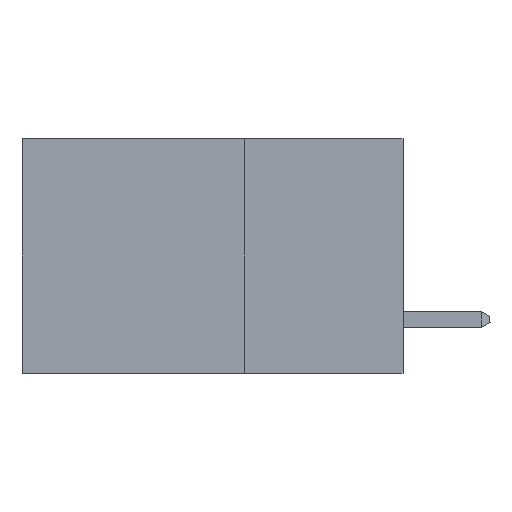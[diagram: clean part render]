
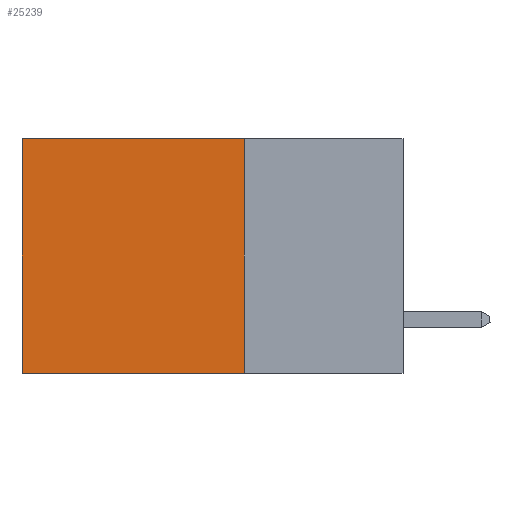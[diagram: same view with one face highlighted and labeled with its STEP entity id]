
A CAD part, left-side view. The second image highlights one B-rep face of the part: STEP entity #25239.
In plain terms, the highlighted planar face has unit normal (-1, 0, 0).
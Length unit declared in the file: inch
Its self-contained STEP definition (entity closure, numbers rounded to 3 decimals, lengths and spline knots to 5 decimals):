
#1947 = CARTESIAN_POINT ( 'NONE',  ( 0.2875, 0.25, 0. ) ) ;
#2857 = DIRECTION ( 'NONE',  ( 0., 1., 0. ) ) ;
#2912 = ORIENTED_EDGE ( 'NONE', *, *, #10901, .F. ) ;
#4572 = VECTOR ( 'NONE', #8543, 39.37008 ) ;
#4784 = VECTOR ( 'NONE', #24970, 39.37008 ) ;
#5266 = VERTEX_POINT ( 'NONE', #1947 ) ;
#7312 = LINE ( 'NONE', #16589, #4784 ) ;
#8152 = EDGE_CURVE ( 'NONE', #25334, #18882, #29301, .T. ) ;
#8543 = DIRECTION ( 'NONE',  ( 0., 0., -1. ) ) ;
#9494 = EDGE_LOOP ( 'NONE', ( #34622, #2912, #14460, #10343 ) ) ;
#10343 = ORIENTED_EDGE ( 'NONE', *, *, #18766, .T. ) ;
#10901 = EDGE_CURVE ( 'NONE', #11568, #18882, #7312, .T. ) ;
#11568 = VERTEX_POINT ( 'NONE', #30639 ) ;
#12068 = DIRECTION ( 'NONE',  ( 0., 0., -1. ) ) ;
#12551 = PLANE ( 'NONE',  #35012 ) ;
#14402 = LINE ( 'NONE', #19249, #26872 ) ;
#14460 = ORIENTED_EDGE ( 'NONE', *, *, #15959, .F. ) ;
#15959 = EDGE_CURVE ( 'NONE', #5266, #11568, #29361, .T. ) ;
#16589 = CARTESIAN_POINT ( 'NONE',  ( 0.2875, 0.25, -0.37 ) ) ;
#17227 = CARTESIAN_POINT ( 'NONE',  ( 0.2875, 0.25, 0. ) ) ;
#17566 = CARTESIAN_POINT ( 'NONE',  ( 0.2875, 0.25, 0. ) ) ;
#17691 = CARTESIAN_POINT ( 'NONE',  ( 0.2875, 0.6, 0. ) ) ;
#18717 = VECTOR ( 'NONE', #33597, 39.37008 ) ;
#18766 = EDGE_CURVE ( 'NONE', #5266, #25334, #14402, .T. ) ;
#18882 = VERTEX_POINT ( 'NONE', #34020 ) ;
#19249 = CARTESIAN_POINT ( 'NONE',  ( 0.2875, 0.25, 0. ) ) ;
#19938 = CARTESIAN_POINT ( 'NONE',  ( 0.2875, 0.6, 0. ) ) ;
#22181 = FACE_OUTER_BOUND ( 'NONE', #9494, .T. ) ;
#24970 = DIRECTION ( 'NONE',  ( 0., 1., 0. ) ) ;
#25239 = ADVANCED_FACE ( 'NONE', ( #22181 ), #12551, .F. ) ;
#25334 = VERTEX_POINT ( 'NONE', #17691 ) ;
#26872 = VECTOR ( 'NONE', #2857, 39.37008 ) ;
#28642 = DIRECTION ( 'NONE',  ( 1., 0., 0. ) ) ;
#29301 = LINE ( 'NONE', #19938, #4572 ) ;
#29361 = LINE ( 'NONE', #17227, #18717 ) ;
#30639 = CARTESIAN_POINT ( 'NONE',  ( 0.2875, 0.25, -0.37 ) ) ;
#33597 = DIRECTION ( 'NONE',  ( 0., 0., -1. ) ) ;
#34020 = CARTESIAN_POINT ( 'NONE',  ( 0.2875, 0.6, -0.37 ) ) ;
#34622 = ORIENTED_EDGE ( 'NONE', *, *, #8152, .T. ) ;
#35012 = AXIS2_PLACEMENT_3D ( 'NONE', #17566, #28642, #12068 ) ;
